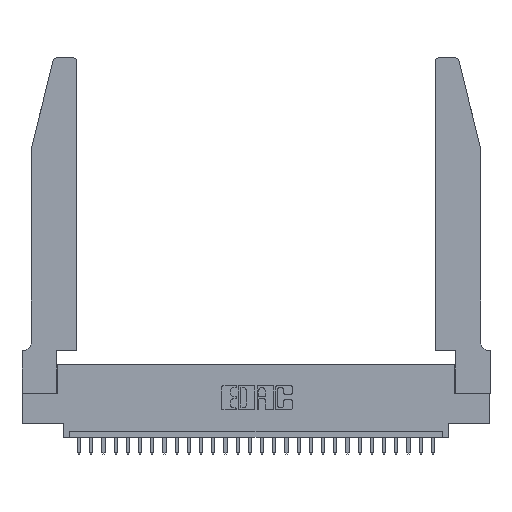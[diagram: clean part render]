
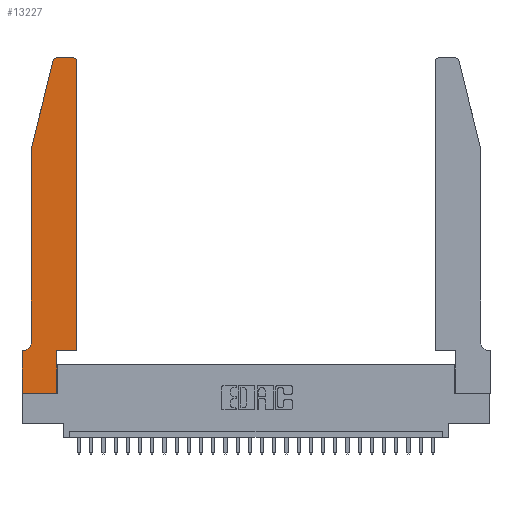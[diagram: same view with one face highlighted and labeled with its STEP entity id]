
A CAD part, top view. The second image highlights one B-rep face of the part: STEP entity #13227.
In plain terms, the highlighted planar face has unit normal (0, 0, 1).
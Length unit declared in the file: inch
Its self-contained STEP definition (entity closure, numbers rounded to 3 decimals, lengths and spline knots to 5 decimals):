
#37 = EDGE_CURVE ( 'NONE', #25120, #28923, #24876, .T. ) ;
#367 = EDGE_CURVE ( 'NONE', #27866, #19878, #9729, .T. ) ;
#564 = ORIENTED_EDGE ( 'NONE', *, *, #11482, .T. ) ;
#1485 = AXIS2_PLACEMENT_3D ( 'NONE', #23728, #28220, #12623 ) ;
#1619 = EDGE_CURVE ( 'NONE', #14627, #26960, #18395, .T. ) ;
#1950 = VERTEX_POINT ( 'NONE', #26896 ) ;
#2195 = CARTESIAN_POINT ( 'NONE',  ( 0.0755, 0.42, 0.37 ) ) ;
#2539 = CARTESIAN_POINT ( 'NONE',  ( 0., 0.35, 0.37 ) ) ;
#2540 = ORIENTED_EDGE ( 'NONE', *, *, #3371, .T. ) ;
#2647 = CARTESIAN_POINT ( 'NONE',  ( 0.4205, 2.72, 0.37 ) ) ;
#3034 = ORIENTED_EDGE ( 'NONE', *, *, #18798, .T. ) ;
#3140 = CARTESIAN_POINT ( 'NONE',  ( 0., 0., 0.37 ) ) ;
#3311 = CARTESIAN_POINT ( 'NONE',  ( 0.2865, 0.35, 0.37 ) ) ;
#3371 = EDGE_CURVE ( 'NONE', #26960, #26241, #25049, .T. ) ;
#3453 = CARTESIAN_POINT ( 'NONE',  ( 0.0755, 2., 0.37 ) ) ;
#3733 = ORIENTED_EDGE ( 'NONE', *, *, #24618, .T. ) ;
#4601 = DIRECTION ( 'NONE',  ( -1., 0., 0. ) ) ;
#4620 = VECTOR ( 'NONE', #4601, 39.37008 ) ;
#4999 = ORIENTED_EDGE ( 'NONE', *, *, #21672, .T. ) ;
#5595 = AXIS2_PLACEMENT_3D ( 'NONE', #2647, #7064, #22805 ) ;
#5759 = DIRECTION ( 'NONE',  ( 0., -1., 0. ) ) ;
#5871 = DIRECTION ( 'NONE',  ( 0., 1., 0. ) ) ;
#5941 = FACE_OUTER_BOUND ( 'NONE', #23577, .T. ) ;
#6054 = CARTESIAN_POINT ( 'NONE',  ( 0.0755, 0.35, 0.37 ) ) ;
#6126 = DIRECTION ( 'NONE',  ( 0., 0., -1. ) ) ;
#6194 = ORIENTED_EDGE ( 'NONE', *, *, #37, .T. ) ;
#6237 = DIRECTION ( 'NONE',  ( 0., 0., 1. ) ) ;
#6471 = CARTESIAN_POINT ( 'NONE',  ( 0.4505, 0.35, 0.37 ) ) ;
#6800 = VERTEX_POINT ( 'NONE', #14754 ) ;
#7064 = DIRECTION ( 'NONE',  ( 0., 0., 1. ) ) ;
#7313 = CARTESIAN_POINT ( 'NONE',  ( 0.0755, 2., 0.37 ) ) ;
#8341 = DIRECTION ( 'NONE',  ( -1., 0., 0. ) ) ;
#8527 = DIRECTION ( 'NONE',  ( 1., 0., 0. ) ) ;
#9192 = ORIENTED_EDGE ( 'NONE', *, *, #1619, .T. ) ;
#9713 = EDGE_CURVE ( 'NONE', #21309, #6800, #15940, .T. ) ;
#9729 = LINE ( 'NONE', #15871, #16373 ) ;
#9863 = VECTOR ( 'NONE', #24421, 39.37008 ) ;
#10986 = VECTOR ( 'NONE', #5871, 39.37008 ) ;
#11482 = EDGE_CURVE ( 'NONE', #19878, #21309, #15155, .T. ) ;
#11572 = CIRCLE ( 'NONE', #1485, 0.03 ) ;
#12429 = CARTESIAN_POINT ( 'NONE',  ( 0.4505, 0.35, 0.37 ) ) ;
#12559 = CARTESIAN_POINT ( 'NONE',  ( 0.0055, 0.35, 0.37 ) ) ;
#12623 = DIRECTION ( 'NONE',  ( 1., 0., 0. ) ) ;
#12781 = ORIENTED_EDGE ( 'NONE', *, *, #24296, .T. ) ;
#13035 = LINE ( 'NONE', #14524, #15803 ) ;
#13227 = ADVANCED_FACE ( 'NONE', ( #5941 ), #28662, .T. ) ;
#13737 = CARTESIAN_POINT ( 'NONE',  ( 0.2865, 0.35, 0.37 ) ) ;
#13773 = LINE ( 'NONE', #20683, #4620 ) ;
#14142 = VERTEX_POINT ( 'NONE', #20858 ) ;
#14380 = LINE ( 'NONE', #25532, #18587 ) ;
#14524 = CARTESIAN_POINT ( 'NONE',  ( 0., 0., 0.37 ) ) ;
#14562 = CIRCLE ( 'NONE', #5595, 0.03 ) ;
#14601 = VECTOR ( 'NONE', #16985, 39.37008 ) ;
#14627 = VERTEX_POINT ( 'NONE', #2195 ) ;
#14754 = CARTESIAN_POINT ( 'NONE',  ( 0.4505, 0.35, 0.37 ) ) ;
#15155 = LINE ( 'NONE', #3311, #10986 ) ;
#15181 = CARTESIAN_POINT ( 'NONE',  ( 0., 0.35, 0.37 ) ) ;
#15803 = VECTOR ( 'NONE', #23689, 39.37008 ) ;
#15842 = VECTOR ( 'NONE', #8341, 39.37008 ) ;
#15871 = CARTESIAN_POINT ( 'NONE',  ( 0., 0., 0.37 ) ) ;
#15940 = LINE ( 'NONE', #12429, #28281 ) ;
#16248 = ORIENTED_EDGE ( 'NONE', *, *, #25267, .T. ) ;
#16373 = VECTOR ( 'NONE', #20416, 39.37008 ) ;
#16797 = DIRECTION ( 'NONE',  ( 1., 0., 0. ) ) ;
#16985 = DIRECTION ( 'NONE',  ( -0.239, -0.971, 0. ) ) ;
#17627 = CARTESIAN_POINT ( 'NONE',  ( 0.2865, 0., 0.37 ) ) ;
#18395 = CIRCLE ( 'NONE', #28219, 0.07 ) ;
#18587 = VECTOR ( 'NONE', #5759, 39.37008 ) ;
#18798 = EDGE_CURVE ( 'NONE', #26241, #27866, #13035, .T. ) ;
#19371 = DIRECTION ( 'NONE',  ( -1., 0., 0. ) ) ;
#19878 = VERTEX_POINT ( 'NONE', #17627 ) ;
#20416 = DIRECTION ( 'NONE',  ( 1., 0., 0. ) ) ;
#20683 = CARTESIAN_POINT ( 'NONE',  ( 0.2605, 2.75, 0.37 ) ) ;
#20858 = CARTESIAN_POINT ( 'NONE',  ( 0.4205, 2.75, 0.37 ) ) ;
#21309 = VERTEX_POINT ( 'NONE', #13737 ) ;
#21672 = EDGE_CURVE ( 'NONE', #1950, #14142, #14562, .T. ) ;
#22805 = DIRECTION ( 'NONE',  ( 1., 0., 0. ) ) ;
#23375 = EDGE_CURVE ( 'NONE', #14142, #27120, #13773, .T. ) ;
#23577 = EDGE_LOOP ( 'NONE', ( #26768, #16248, #6194, #3733, #9192, #2540, #3034, #26530, #564, #27065, #12781, #4999 ) ) ;
#23689 = DIRECTION ( 'NONE',  ( 0., -1., 0. ) ) ;
#23728 = CARTESIAN_POINT ( 'NONE',  ( 0.284, 2.72, 0.37 ) ) ;
#24296 = EDGE_CURVE ( 'NONE', #6800, #1950, #26429, .T. ) ;
#24421 = DIRECTION ( 'NONE',  ( 0., 1., 0. ) ) ;
#24618 = EDGE_CURVE ( 'NONE', #28923, #14627, #14380, .T. ) ;
#24764 = CARTESIAN_POINT ( 'NONE',  ( 0.284, 2.75, 0.37 ) ) ;
#24876 = LINE ( 'NONE', #3453, #14601 ) ;
#25049 = LINE ( 'NONE', #6054, #15842 ) ;
#25120 = VERTEX_POINT ( 'NONE', #25306 ) ;
#25267 = EDGE_CURVE ( 'NONE', #27120, #25120, #11572, .T. ) ;
#25306 = CARTESIAN_POINT ( 'NONE',  ( 0.25487, 2.72718, 0.37 ) ) ;
#25532 = CARTESIAN_POINT ( 'NONE',  ( 0.0755, 2., 0.37 ) ) ;
#26241 = VERTEX_POINT ( 'NONE', #2539 ) ;
#26429 = LINE ( 'NONE', #6471, #9863 ) ;
#26530 = ORIENTED_EDGE ( 'NONE', *, *, #367, .T. ) ;
#26768 = ORIENTED_EDGE ( 'NONE', *, *, #23375, .T. ) ;
#26896 = CARTESIAN_POINT ( 'NONE',  ( 0.4505, 2.72, 0.37 ) ) ;
#26960 = VERTEX_POINT ( 'NONE', #12559 ) ;
#27065 = ORIENTED_EDGE ( 'NONE', *, *, #9713, .T. ) ;
#27120 = VERTEX_POINT ( 'NONE', #24764 ) ;
#27150 = AXIS2_PLACEMENT_3D ( 'NONE', #15181, #6237, #8527 ) ;
#27866 = VERTEX_POINT ( 'NONE', #3140 ) ;
#28219 = AXIS2_PLACEMENT_3D ( 'NONE', #28433, #6126, #19371 ) ;
#28220 = DIRECTION ( 'NONE',  ( 0., 0., 1. ) ) ;
#28281 = VECTOR ( 'NONE', #16797, 39.37008 ) ;
#28433 = CARTESIAN_POINT ( 'NONE',  ( 0.0055, 0.42, 0.37 ) ) ;
#28662 = PLANE ( 'NONE',  #27150 ) ;
#28923 = VERTEX_POINT ( 'NONE', #7313 ) ;
